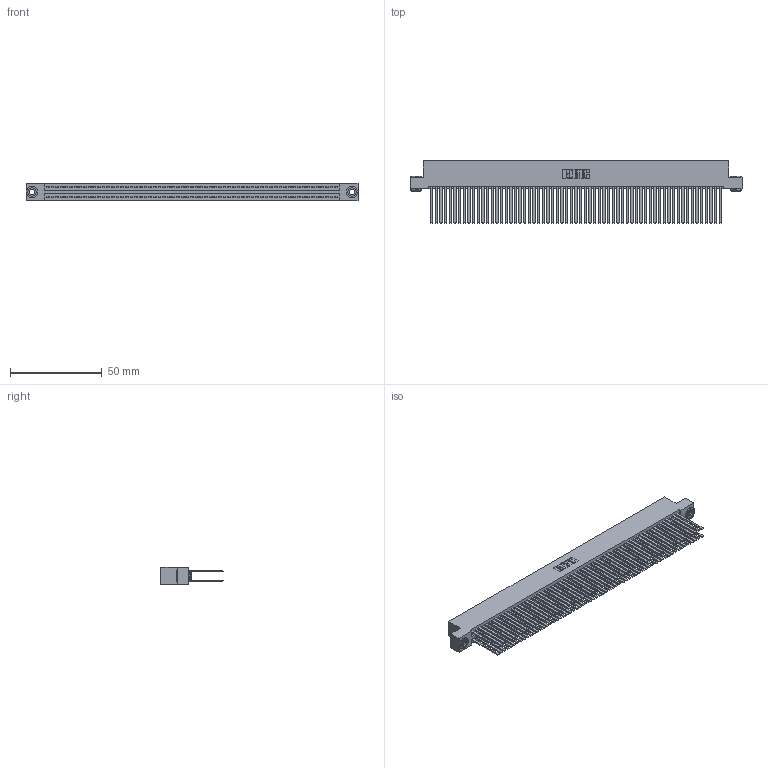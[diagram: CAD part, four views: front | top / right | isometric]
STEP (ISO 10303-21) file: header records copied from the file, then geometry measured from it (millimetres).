
FILE_DESCRIPTION (( 'STEP AP203' ), '1' );
FILE_NAME ('395-126-544-203.STEP', '2018-12-04T06:06:33', ( '' ), ( '' ), 'SwSTEP 2.0', 'SolidWorks 2016', '' );
FILE_SCHEMA (( 'CONFIG_CONTROL_DESIGN' ));
Length unit declared in the file: inch
Products named in the file (4): 345-250-002_345-250-002-102; 345-292-001_345-293-144; 345 Part_Flush Mounting Lugs - 0.156 Dia-TH; 395-126-544-203
Assembly tree (129 placements, depth 2):
  395-126-544-203
    345 Part_Flush Mounting Lugs - 0.156 Dia-TH
    345-292-001_345-293-144  x126
    345-250-002_345-250-002-102  x2
Bounding box: 181.23 x 33.96 x 9.4 mm (x, y, z)
Volume: 19585.4 mm3; surface area: 34738.9 mm2
Topology: 129 solids, 129 shells, 5708 faces, 16923 edges, 11110 vertices
Faces by surface type: plane 3744, cylinder 1956, cone 8
Entity records: 47070 total; most frequent: CARTESIAN_POINT 7843, ORIENTED_EDGE 7770, DIRECTION 6919, EDGE_CURVE 3885, VECTOR 3481, LINE 3481, VERTEX_POINT 2586, AXIS2_PLACEMENT_3D 1719
